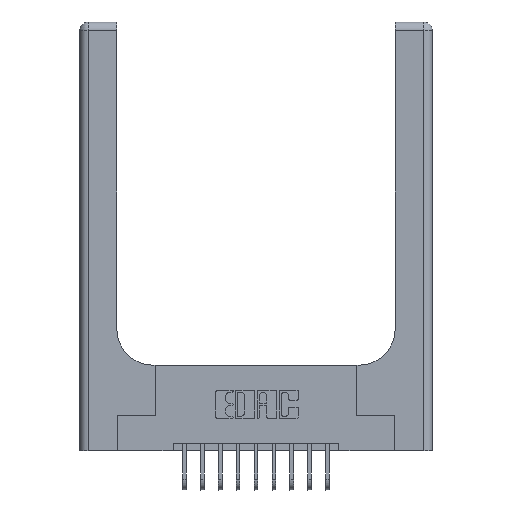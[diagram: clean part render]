
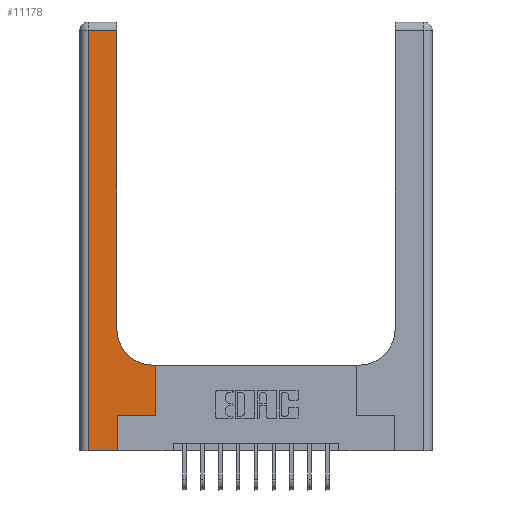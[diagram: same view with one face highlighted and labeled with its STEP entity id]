
A CAD part, top view. The second image highlights one B-rep face of the part: STEP entity #11178.
In plain terms, the highlighted planar face has unit normal (0, 0, 1).
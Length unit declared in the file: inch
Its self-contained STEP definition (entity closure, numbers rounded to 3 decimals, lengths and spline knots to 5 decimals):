
#119 = VECTOR ( 'NONE', #2134, 39.37008 ) ;
#297 = DIRECTION ( 'NONE',  ( 0., 1., 0. ) ) ;
#835 = DIRECTION ( 'NONE',  ( 0., 1., 0. ) ) ;
#875 = CARTESIAN_POINT ( 'NONE',  ( 0.51, 0.85, 0.37 ) ) ;
#1127 = ORIENTED_EDGE ( 'NONE', *, *, #7335, .T. ) ;
#1318 = VERTEX_POINT ( 'NONE', #12891 ) ;
#1524 = EDGE_CURVE ( 'NONE', #15992, #16616, #11894, .T. ) ;
#1805 = CARTESIAN_POINT ( 'NONE',  ( 0.51, 0.6, 0.37 ) ) ;
#2051 = CARTESIAN_POINT ( 'NONE',  ( 0.26, 2.94, 0.37 ) ) ;
#2134 = DIRECTION ( 'NONE',  ( -1., 0., 0. ) ) ;
#2221 = LINE ( 'NONE', #17111, #119 ) ;
#2223 = DIRECTION ( 'NONE',  ( 0., 0., -1. ) ) ;
#2311 = DIRECTION ( 'NONE',  ( 1., 0., 0. ) ) ;
#2905 = CARTESIAN_POINT ( 'NONE',  ( 0.26, 3., 0.37 ) ) ;
#3178 = EDGE_CURVE ( 'NONE', #17599, #13477, #7382, .T. ) ;
#3351 = ORIENTED_EDGE ( 'NONE', *, *, #4246, .T. ) ;
#3670 = VERTEX_POINT ( 'NONE', #11397 ) ;
#3893 = DIRECTION ( 'NONE',  ( 0., -1., 0. ) ) ;
#4246 = EDGE_CURVE ( 'NONE', #16035, #15998, #16653, .T. ) ;
#4499 = CARTESIAN_POINT ( 'NONE',  ( 0.26, 0.85, 0.37 ) ) ;
#4717 = DIRECTION ( 'NONE',  ( -1., 0., 0. ) ) ;
#4939 = ORIENTED_EDGE ( 'NONE', *, *, #3178, .T. ) ;
#5123 = DIRECTION ( 'NONE',  ( 1., 0., 0. ) ) ;
#5184 = EDGE_LOOP ( 'NONE', ( #9451, #13409, #17045, #1127, #4939, #9982, #15604, #14167, #3351 ) ) ;
#5224 = CARTESIAN_POINT ( 'NONE',  ( 0.06, 3., 0.37 ) ) ;
#5330 = CARTESIAN_POINT ( 'NONE',  ( 0.528, 0.25, 0.37 ) ) ;
#6021 = VECTOR ( 'NONE', #4717, 39.37008 ) ;
#6045 = VECTOR ( 'NONE', #3893, 39.37008 ) ;
#6592 = VECTOR ( 'NONE', #16981, 39.37008 ) ;
#6692 = LINE ( 'NONE', #5330, #7450 ) ;
#6930 = LINE ( 'NONE', #8009, #9345 ) ;
#6994 = VECTOR ( 'NONE', #2311, 39.37008 ) ;
#7034 = LINE ( 'NONE', #2905, #14781 ) ;
#7201 = EDGE_CURVE ( 'NONE', #14089, #16035, #2221, .T. ) ;
#7335 = EDGE_CURVE ( 'NONE', #1318, #17599, #14683, .T. ) ;
#7382 = LINE ( 'NONE', #12600, #6592 ) ;
#7450 = VECTOR ( 'NONE', #835, 39.37008 ) ;
#7529 = DIRECTION ( 'NONE',  ( 0., 0., -1. ) ) ;
#7702 = PLANE ( 'NONE',  #11765 ) ;
#8009 = CARTESIAN_POINT ( 'NONE',  ( 0.265, 0.25, 0.37 ) ) ;
#8969 = CARTESIAN_POINT ( 'NONE',  ( 0., 3., 0.37 ) ) ;
#9345 = VECTOR ( 'NONE', #5123, 39.37008 ) ;
#9416 = CARTESIAN_POINT ( 'NONE',  ( 0.265, 0.25, 0.37 ) ) ;
#9451 = ORIENTED_EDGE ( 'NONE', *, *, #15404, .T. ) ;
#9982 = ORIENTED_EDGE ( 'NONE', *, *, #17345, .T. ) ;
#10407 = EDGE_CURVE ( 'NONE', #3670, #14089, #6692, .T. ) ;
#10520 = LINE ( 'NONE', #5224, #6045 ) ;
#11178 = ADVANCED_FACE ( 'NONE', ( #11746 ), #7702, .F. ) ;
#11397 = CARTESIAN_POINT ( 'NONE',  ( 0.528, 0.25, 0.37 ) ) ;
#11746 = FACE_OUTER_BOUND ( 'NONE', #5184, .T. ) ;
#11765 = AXIS2_PLACEMENT_3D ( 'NONE', #8969, #7529, #12995 ) ;
#11894 = LINE ( 'NONE', #17360, #6021 ) ;
#11946 = EDGE_CURVE ( 'NONE', #16616, #1318, #10520, .T. ) ;
#12157 = CARTESIAN_POINT ( 'NONE',  ( 0.528, 0.6, 0.37 ) ) ;
#12600 = CARTESIAN_POINT ( 'NONE',  ( 0.265, 0., 0.37 ) ) ;
#12891 = CARTESIAN_POINT ( 'NONE',  ( 0.06, 0., 0.37 ) ) ;
#12995 = DIRECTION ( 'NONE',  ( -1., 0., 0. ) ) ;
#13245 = CARTESIAN_POINT ( 'NONE',  ( 0.265, 0., 0.37 ) ) ;
#13409 = ORIENTED_EDGE ( 'NONE', *, *, #1524, .T. ) ;
#13477 = VERTEX_POINT ( 'NONE', #9416 ) ;
#13768 = CARTESIAN_POINT ( 'NONE',  ( 0.06, 2.94, 0.37 ) ) ;
#14089 = VERTEX_POINT ( 'NONE', #12157 ) ;
#14167 = ORIENTED_EDGE ( 'NONE', *, *, #7201, .T. ) ;
#14683 = LINE ( 'NONE', #14951, #6994 ) ;
#14781 = VECTOR ( 'NONE', #297, 39.37008 ) ;
#14951 = CARTESIAN_POINT ( 'NONE',  ( 0., 0., 0.37 ) ) ;
#15404 = EDGE_CURVE ( 'NONE', #15998, #15992, #7034, .T. ) ;
#15604 = ORIENTED_EDGE ( 'NONE', *, *, #10407, .T. ) ;
#15954 = DIRECTION ( 'NONE',  ( 1., 0., 0. ) ) ;
#15992 = VERTEX_POINT ( 'NONE', #2051 ) ;
#15998 = VERTEX_POINT ( 'NONE', #4499 ) ;
#16035 = VERTEX_POINT ( 'NONE', #1805 ) ;
#16081 = AXIS2_PLACEMENT_3D ( 'NONE', #875, #2223, #15954 ) ;
#16616 = VERTEX_POINT ( 'NONE', #13768 ) ;
#16653 = CIRCLE ( 'NONE', #16081, 0.25 ) ;
#16981 = DIRECTION ( 'NONE',  ( 0., 1., 0. ) ) ;
#17045 = ORIENTED_EDGE ( 'NONE', *, *, #11946, .T. ) ;
#17111 = CARTESIAN_POINT ( 'NONE',  ( 0.26, 0.6, 0.37 ) ) ;
#17345 = EDGE_CURVE ( 'NONE', #13477, #3670, #6930, .T. ) ;
#17360 = CARTESIAN_POINT ( 'NONE',  ( 0., 2.94, 0.37 ) ) ;
#17599 = VERTEX_POINT ( 'NONE', #13245 ) ;
